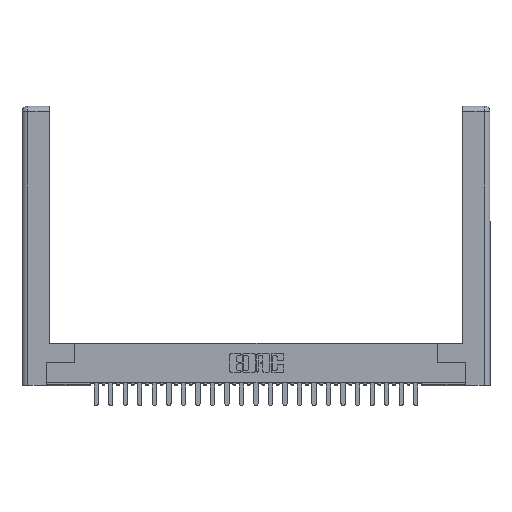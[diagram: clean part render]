
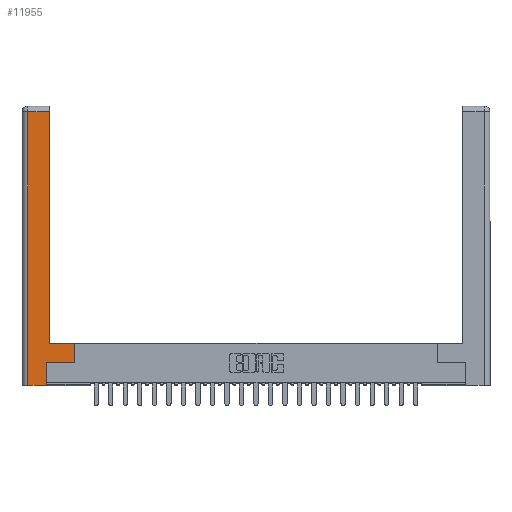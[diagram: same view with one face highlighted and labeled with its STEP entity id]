
A CAD part, top view. The second image highlights one B-rep face of the part: STEP entity #11955.
In plain terms, the highlighted planar face has unit normal (0, 0, 1).
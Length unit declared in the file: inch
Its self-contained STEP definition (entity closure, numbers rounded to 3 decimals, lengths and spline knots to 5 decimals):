
#216 = CARTESIAN_POINT ( 'NONE',  ( 0., 0., 0. ) ) ;
#313 = DIRECTION ( 'NONE',  ( -1., 0., 0. ) ) ;
#808 = EDGE_CURVE ( 'NONE', #2010, #14015, #5774, .T. ) ;
#1169 = CARTESIAN_POINT ( 'NONE',  ( 0.0615, 2.94, 0. ) ) ;
#1588 = VERTEX_POINT ( 'NONE', #13859 ) ;
#2010 = VERTEX_POINT ( 'NONE', #1169 ) ;
#2519 = ORIENTED_EDGE ( 'NONE', *, *, #808, .T. ) ;
#2899 = ORIENTED_EDGE ( 'NONE', *, *, #4482, .T. ) ;
#3250 = ORIENTED_EDGE ( 'NONE', *, *, #24146, .T. ) ;
#4482 = EDGE_CURVE ( 'NONE', #1588, #12791, #28542, .T. ) ;
#4663 = CARTESIAN_POINT ( 'NONE',  ( 0.265, 0.245, 0. ) ) ;
#4699 = DIRECTION ( 'NONE',  ( 0., 1., 0. ) ) ;
#4707 = CARTESIAN_POINT ( 'NONE',  ( 0.295, 2.94, 0. ) ) ;
#5248 = EDGE_LOOP ( 'NONE', ( #26663, #3250, #2519, #15674, #15276, #20722, #2899, #8730 ) ) ;
#5603 = EDGE_CURVE ( 'NONE', #14015, #12362, #23129, .T. ) ;
#5774 = LINE ( 'NONE', #8508, #15897 ) ;
#6443 = VERTEX_POINT ( 'NONE', #4663 ) ;
#6515 = LINE ( 'NONE', #16084, #25928 ) ;
#7250 = VECTOR ( 'NONE', #15345, 39.37008 ) ;
#7971 = CARTESIAN_POINT ( 'NONE',  ( 0.265, 0., 0. ) ) ;
#8508 = CARTESIAN_POINT ( 'NONE',  ( 0.0615, 0., 0. ) ) ;
#8730 = ORIENTED_EDGE ( 'NONE', *, *, #22254, .T. ) ;
#9101 = CARTESIAN_POINT ( 'NONE',  ( 0.565, 0.45, 0. ) ) ;
#9152 = CARTESIAN_POINT ( 'NONE',  ( 0.295, 3., 0. ) ) ;
#9386 = CARTESIAN_POINT ( 'NONE',  ( 0.0615, 0., 0. ) ) ;
#10286 = DIRECTION ( 'NONE',  ( -1., 0., 0. ) ) ;
#10519 = LINE ( 'NONE', #20063, #7250 ) ;
#11249 = VECTOR ( 'NONE', #15791, 39.37008 ) ;
#11313 = CARTESIAN_POINT ( 'NONE',  ( 0.565, 0.45, 0. ) ) ;
#11955 = ADVANCED_FACE ( 'NONE', ( #21384 ), #25520, .F. ) ;
#12197 = VECTOR ( 'NONE', #10286, 39.37008 ) ;
#12362 = VERTEX_POINT ( 'NONE', #7971 ) ;
#12389 = CARTESIAN_POINT ( 'NONE',  ( 0.0615, 2.94, 0. ) ) ;
#12470 = VERTEX_POINT ( 'NONE', #22146 ) ;
#12791 = VERTEX_POINT ( 'NONE', #9101 ) ;
#13612 = DIRECTION ( 'NONE',  ( 0., 1., 0. ) ) ;
#13859 = CARTESIAN_POINT ( 'NONE',  ( 0.565, 0.245, 0. ) ) ;
#14015 = VERTEX_POINT ( 'NONE', #9386 ) ;
#15276 = ORIENTED_EDGE ( 'NONE', *, *, #18215, .T. ) ;
#15345 = DIRECTION ( 'NONE',  ( 0., 1., 0. ) ) ;
#15674 = ORIENTED_EDGE ( 'NONE', *, *, #5603, .T. ) ;
#15791 = DIRECTION ( 'NONE',  ( 1., 0., 0. ) ) ;
#15897 = VECTOR ( 'NONE', #27118, 39.37008 ) ;
#16084 = CARTESIAN_POINT ( 'NONE',  ( 0.295, 0.45, 0. ) ) ;
#18215 = EDGE_CURVE ( 'NONE', #12362, #6443, #10519, .T. ) ;
#18398 = DIRECTION ( 'NONE',  ( -1., 0., 0. ) ) ;
#19108 = CARTESIAN_POINT ( 'NONE',  ( 0.265, 0., 0. ) ) ;
#19791 = EDGE_CURVE ( 'NONE', #12470, #29170, #28525, .T. ) ;
#20063 = CARTESIAN_POINT ( 'NONE',  ( 0.265, 0.245, 0. ) ) ;
#20562 = LINE ( 'NONE', #29639, #11249 ) ;
#20652 = VECTOR ( 'NONE', #13612, 39.37008 ) ;
#20722 = ORIENTED_EDGE ( 'NONE', *, *, #22087, .T. ) ;
#21384 = FACE_OUTER_BOUND ( 'NONE', #5248, .T. ) ;
#22087 = EDGE_CURVE ( 'NONE', #6443, #1588, #20562, .T. ) ;
#22146 = CARTESIAN_POINT ( 'NONE',  ( 0.295, 0.45, 0. ) ) ;
#22254 = EDGE_CURVE ( 'NONE', #12791, #12470, #6515, .T. ) ;
#23129 = LINE ( 'NONE', #19108, #29256 ) ;
#23347 = LINE ( 'NONE', #12389, #12197 ) ;
#23678 = AXIS2_PLACEMENT_3D ( 'NONE', #216, #27793, #313 ) ;
#24146 = EDGE_CURVE ( 'NONE', #29170, #2010, #23347, .T. ) ;
#25520 = PLANE ( 'NONE',  #23678 ) ;
#25928 = VECTOR ( 'NONE', #18398, 39.37008 ) ;
#26045 = DIRECTION ( 'NONE',  ( 1., 0., 0. ) ) ;
#26663 = ORIENTED_EDGE ( 'NONE', *, *, #19791, .T. ) ;
#27118 = DIRECTION ( 'NONE',  ( 0., -1., 0. ) ) ;
#27793 = DIRECTION ( 'NONE',  ( 0., 0., -1. ) ) ;
#28525 = LINE ( 'NONE', #9152, #29614 ) ;
#28542 = LINE ( 'NONE', #11313, #20652 ) ;
#29170 = VERTEX_POINT ( 'NONE', #4707 ) ;
#29256 = VECTOR ( 'NONE', #26045, 39.37008 ) ;
#29614 = VECTOR ( 'NONE', #4699, 39.37008 ) ;
#29639 = CARTESIAN_POINT ( 'NONE',  ( 0.565, 0.245, 0. ) ) ;
